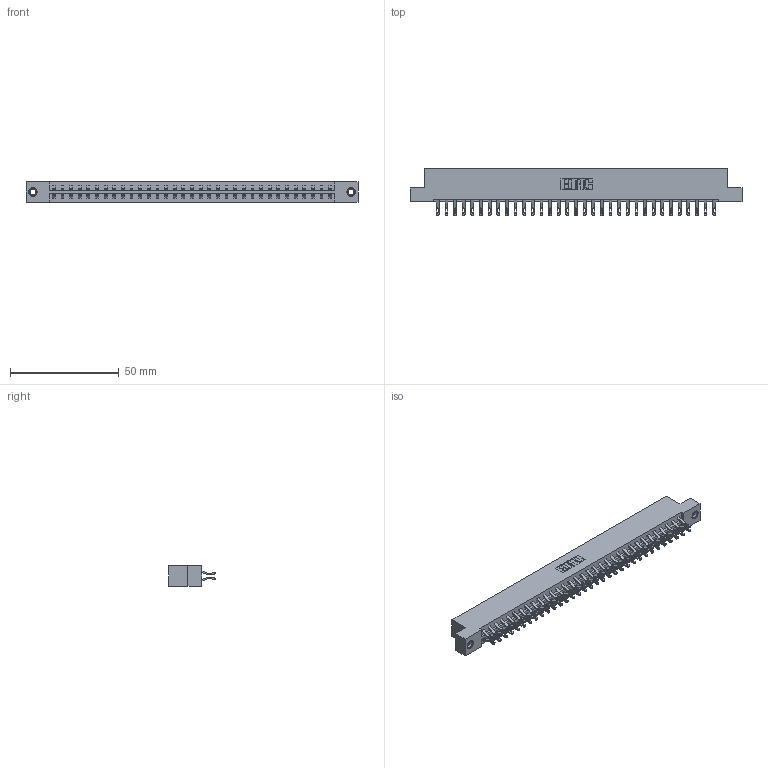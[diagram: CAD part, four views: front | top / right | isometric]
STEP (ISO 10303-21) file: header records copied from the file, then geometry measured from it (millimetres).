
FILE_DESCRIPTION (( 'STEP AP203' ), '1' );
FILE_NAME ('333-066-555-207.STEP', '2018-08-04T11:47:35', ( '' ), ( '' ), 'SwSTEP 2.0', 'SolidWorks 2016', '' );
FILE_SCHEMA (( 'CONFIG_CONTROL_DESIGN' ));
Length unit declared in the file: inch
Products named in the file (4): 333 Part_Flush - .156 Dia - TI; 345-292-001_555 Tail; 345-250-001_345-250-005-103; 333-066-555-207
Assembly tree (69 placements, depth 2):
  333-066-555-207
    333 Part_Flush - .156 Dia - TI
    345-292-001_555 Tail  x66
    345-250-001_345-250-005-103  x2
Bounding box: 152.3 x 21.47 x 9.4 mm (x, y, z)
Volume: 15642.6 mm3; surface area: 19146.7 mm2
Topology: 69 solids, 69 shells, 4002 faces, 12525 edges, 8342 vertices
Faces by surface type: plane 2346, cylinder 1640, cone 12, torus 4
Entity records: 23906 total; most frequent: CARTESIAN_POINT 3991, ORIENTED_EDGE 3890, DIRECTION 3427, EDGE_CURVE 1945, LINE 1777, VECTOR 1777, VERTEX_POINT 1292, AXIS2_PLACEMENT_3D 825
